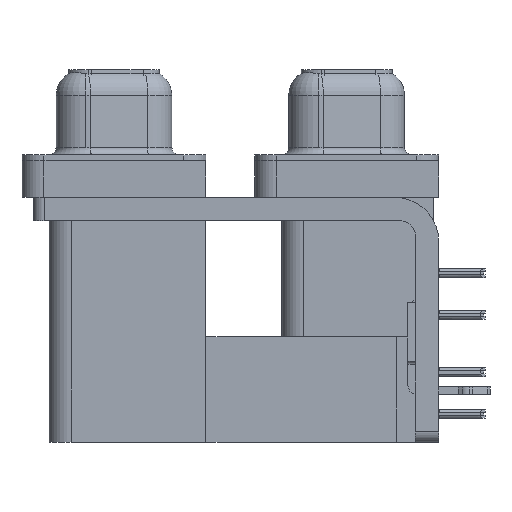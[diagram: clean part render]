
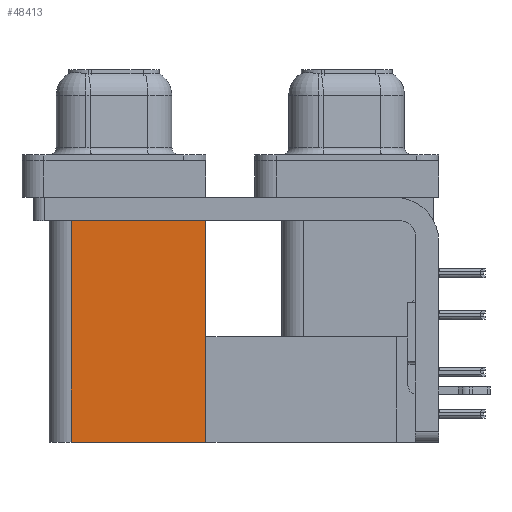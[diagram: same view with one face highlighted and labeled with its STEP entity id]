
A CAD part, left-side view. The second image highlights one B-rep face of the part: STEP entity #48413.
In plain terms, the highlighted planar face has unit normal (-1, 0, 0).
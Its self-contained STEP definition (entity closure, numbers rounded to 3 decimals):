
#1356 = LINE ( 'NONE', #43671, #43494 ) ;
#2860 = DIRECTION ( 'NONE',  ( 1., 0., 0. ) ) ;
#3013 = LINE ( 'NONE', #5847, #37065 ) ;
#4524 = CARTESIAN_POINT ( 'NONE',  ( 3.765, 18.8, -19.2 ) ) ;
#5381 = DIRECTION ( 'NONE',  ( 0., 1., 0. ) ) ;
#5847 = CARTESIAN_POINT ( 'NONE',  ( 3.765, 9.6, -19.2 ) ) ;
#6207 = FACE_OUTER_BOUND ( 'NONE', #12338, .T. ) ;
#6323 = LINE ( 'NONE', #4524, #29137 ) ;
#6410 = CARTESIAN_POINT ( 'NONE',  ( 3.765, 9.6, -19.2 ) ) ;
#6691 = CARTESIAN_POINT ( 'NONE',  ( 3.765, 9.6, -19.2 ) ) ;
#9881 = ORIENTED_EDGE ( 'NONE', *, *, #31033, .T. ) ;
#12338 = EDGE_LOOP ( 'NONE', ( #9881, #18063, #41032, #47262 ) ) ;
#18063 = ORIENTED_EDGE ( 'NONE', *, *, #43893, .F. ) ;
#20575 = VERTEX_POINT ( 'NONE', #34676 ) ;
#21778 = CARTESIAN_POINT ( 'NONE',  ( 3.765, 9.6, -19.2 ) ) ;
#22459 = VERTEX_POINT ( 'NONE', #22826 ) ;
#22826 = CARTESIAN_POINT ( 'NONE',  ( 3.765, 9.6, -2.5 ) ) ;
#24882 = CARTESIAN_POINT ( 'NONE',  ( 3.765, 18.8, -19.2 ) ) ;
#29137 = VECTOR ( 'NONE', #47826, 1000. ) ;
#29437 = DIRECTION ( 'NONE',  ( 0., 0., 1. ) ) ;
#31033 = EDGE_CURVE ( 'NONE', #22459, #20575, #1356, .T. ) ;
#33121 = PLANE ( 'NONE',  #44279 ) ;
#34676 = CARTESIAN_POINT ( 'NONE',  ( 3.765, 18.8, -2.5 ) ) ;
#37065 = VECTOR ( 'NONE', #29437, 1000. ) ;
#38151 = EDGE_CURVE ( 'NONE', #40222, #22459, #3013, .T. ) ;
#38511 = VECTOR ( 'NONE', #5381, 1000. ) ;
#40222 = VERTEX_POINT ( 'NONE', #6410 ) ;
#41032 = ORIENTED_EDGE ( 'NONE', *, *, #47677, .F. ) ;
#41813 = DIRECTION ( 'NONE',  ( 0., 0., -1. ) ) ;
#43442 = VERTEX_POINT ( 'NONE', #24882 ) ;
#43494 = VECTOR ( 'NONE', #47489, 1000. ) ;
#43671 = CARTESIAN_POINT ( 'NONE',  ( 3.765, 9.6, -2.5 ) ) ;
#43893 = EDGE_CURVE ( 'NONE', #43442, #20575, #6323, .T. ) ;
#44279 = AXIS2_PLACEMENT_3D ( 'NONE', #6691, #2860, #41813 ) ;
#45340 = LINE ( 'NONE', #21778, #38511 ) ;
#47262 = ORIENTED_EDGE ( 'NONE', *, *, #38151, .T. ) ;
#47489 = DIRECTION ( 'NONE',  ( 0., 1., 0. ) ) ;
#47677 = EDGE_CURVE ( 'NONE', #40222, #43442, #45340, .T. ) ;
#47826 = DIRECTION ( 'NONE',  ( 0., 0., 1. ) ) ;
#48413 = ADVANCED_FACE ( 'NONE', ( #6207 ), #33121, .F. ) ;
